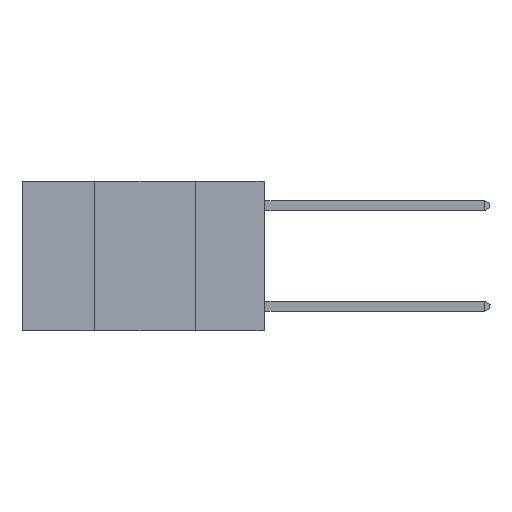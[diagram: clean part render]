
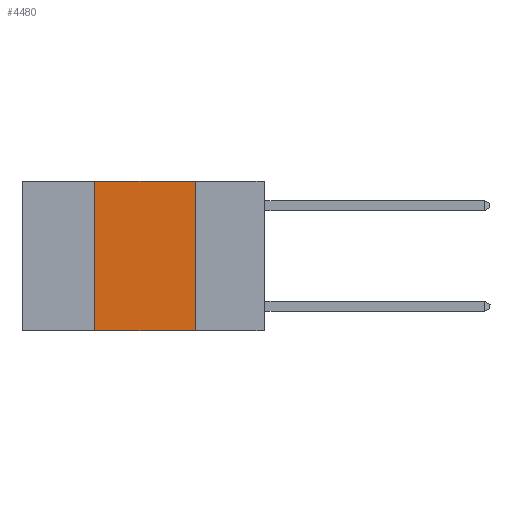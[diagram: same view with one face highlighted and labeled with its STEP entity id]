
A CAD part, left-side view. The second image highlights one B-rep face of the part: STEP entity #4480.
In plain terms, the highlighted planar face has unit normal (-1, 0, 0).
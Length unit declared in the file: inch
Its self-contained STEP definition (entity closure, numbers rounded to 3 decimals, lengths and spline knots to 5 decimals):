
#168 = ORIENTED_EDGE ( 'NONE', *, *, #8826, .F. ) ;
#331 = CARTESIAN_POINT ( 'NONE',  ( 0., 0.42, -0.37 ) ) ;
#334 = CARTESIAN_POINT ( 'NONE',  ( 0., 0.17, -0.37 ) ) ;
#349 = VERTEX_POINT ( 'NONE', #334 ) ;
#457 = VERTEX_POINT ( 'NONE', #331 ) ;
#1169 = LINE ( 'NONE', #6645, #8737 ) ;
#1426 = LINE ( 'NONE', #8460, #3500 ) ;
#1955 = CARTESIAN_POINT ( 'NONE',  ( 0., 0.42, 0. ) ) ;
#2246 = DIRECTION ( 'NONE',  ( 0., -1., 0. ) ) ;
#2446 = ORIENTED_EDGE ( 'NONE', *, *, #5477, .F. ) ;
#2495 = CARTESIAN_POINT ( 'NONE',  ( 0., 0.6, -0.37 ) ) ;
#3183 = VERTEX_POINT ( 'NONE', #4450 ) ;
#3269 = LINE ( 'NONE', #4281, #7140 ) ;
#3353 = EDGE_LOOP ( 'NONE', ( #2446, #168, #8423, #4377 ) ) ;
#3500 = VECTOR ( 'NONE', #9131, 39.37008 ) ;
#3780 = FACE_OUTER_BOUND ( 'NONE', #3353, .T. ) ;
#4281 = CARTESIAN_POINT ( 'NONE',  ( 0., 0.42, 0. ) ) ;
#4377 = ORIENTED_EDGE ( 'NONE', *, *, #5807, .T. ) ;
#4444 = AXIS2_PLACEMENT_3D ( 'NONE', #9283, #8871, #8736 ) ;
#4450 = CARTESIAN_POINT ( 'NONE',  ( 0., 0.17, 0. ) ) ;
#4480 = ADVANCED_FACE ( 'NONE', ( #3780 ), #8917, .F. ) ;
#5027 = DIRECTION ( 'NONE',  ( 0., 0., 1. ) ) ;
#5183 = VECTOR ( 'NONE', #2246, 39.37008 ) ;
#5477 = EDGE_CURVE ( 'NONE', #3183, #349, #1169, .T. ) ;
#5807 = EDGE_CURVE ( 'NONE', #457, #349, #7260, .T. ) ;
#6203 = EDGE_CURVE ( 'NONE', #457, #8059, #3269, .T. ) ;
#6450 = DIRECTION ( 'NONE',  ( 0., 0., -1. ) ) ;
#6645 = CARTESIAN_POINT ( 'NONE',  ( 0., 0.17, 0. ) ) ;
#7140 = VECTOR ( 'NONE', #5027, 39.37008 ) ;
#7260 = LINE ( 'NONE', #2495, #5183 ) ;
#8059 = VERTEX_POINT ( 'NONE', #1955 ) ;
#8423 = ORIENTED_EDGE ( 'NONE', *, *, #6203, .F. ) ;
#8460 = CARTESIAN_POINT ( 'NONE',  ( 0., 0.6, 0. ) ) ;
#8736 = DIRECTION ( 'NONE',  ( 0., 0., -1. ) ) ;
#8737 = VECTOR ( 'NONE', #6450, 39.37008 ) ;
#8826 = EDGE_CURVE ( 'NONE', #8059, #3183, #1426, .T. ) ;
#8871 = DIRECTION ( 'NONE',  ( 1., 0., 0. ) ) ;
#8917 = PLANE ( 'NONE',  #4444 ) ;
#9131 = DIRECTION ( 'NONE',  ( 0., -1., 0. ) ) ;
#9283 = CARTESIAN_POINT ( 'NONE',  ( 0., 0.6, 0. ) ) ;
